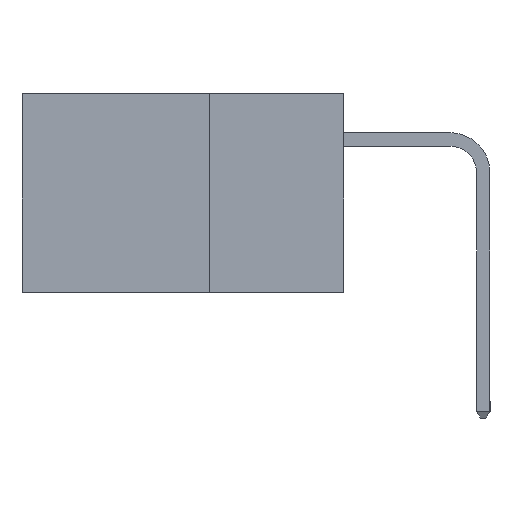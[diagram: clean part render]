
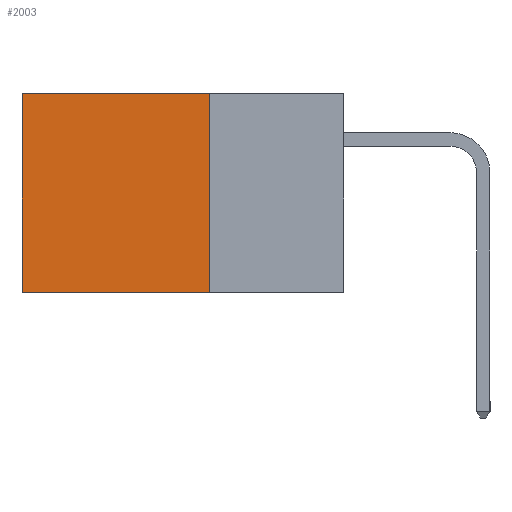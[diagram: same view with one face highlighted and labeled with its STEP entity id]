
A CAD part, left-side view. The second image highlights one B-rep face of the part: STEP entity #2003.
In plain terms, the highlighted planar face has unit normal (-1, 0, 0).
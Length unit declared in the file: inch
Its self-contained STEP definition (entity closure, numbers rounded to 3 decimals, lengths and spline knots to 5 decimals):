
#480 = VECTOR ( 'NONE', #2758, 39.37008 ) ;
#621 = CARTESIAN_POINT ( 'NONE',  ( 0.2615, 0.25, -0.37 ) ) ;
#810 = LINE ( 'NONE', #5589, #8700 ) ;
#1602 = EDGE_CURVE ( 'NONE', #5127, #11629, #3533, .T. ) ;
#2003 = ADVANCED_FACE ( 'NONE', ( #2388 ), #10919, .F. ) ;
#2063 = CARTESIAN_POINT ( 'NONE',  ( 0.2615, 0.25, 0. ) ) ;
#2388 = FACE_OUTER_BOUND ( 'NONE', #12728, .T. ) ;
#2590 = VERTEX_POINT ( 'NONE', #5535 ) ;
#2758 = DIRECTION ( 'NONE',  ( 0., 0., -1. ) ) ;
#3533 = LINE ( 'NONE', #10657, #480 ) ;
#5127 = VERTEX_POINT ( 'NONE', #14093 ) ;
#5492 = LINE ( 'NONE', #2063, #12486 ) ;
#5535 = CARTESIAN_POINT ( 'NONE',  ( 0.2615, 0.6, 0. ) ) ;
#5589 = CARTESIAN_POINT ( 'NONE',  ( 0.2615, 0.25, -0.37 ) ) ;
#5683 = ORIENTED_EDGE ( 'NONE', *, *, #10510, .T. ) ;
#6492 = CARTESIAN_POINT ( 'NONE',  ( 0.2615, 0.25, -0.37 ) ) ;
#6732 = DIRECTION ( 'NONE',  ( 0., 1., 0. ) ) ;
#7025 = DIRECTION ( 'NONE',  ( 0., 0., -1. ) ) ;
#7099 = DIRECTION ( 'NONE',  ( 1., 0., 0. ) ) ;
#7824 = ORIENTED_EDGE ( 'NONE', *, *, #10546, .F. ) ;
#8700 = VECTOR ( 'NONE', #10100, 39.37008 ) ;
#8756 = ORIENTED_EDGE ( 'NONE', *, *, #9602, .T. ) ;
#9108 = LINE ( 'NONE', #11697, #14690 ) ;
#9436 = DIRECTION ( 'NONE',  ( 0., 0., -1. ) ) ;
#9602 = EDGE_CURVE ( 'NONE', #2590, #11001, #9108, .T. ) ;
#10100 = DIRECTION ( 'NONE',  ( 0., 1., 0. ) ) ;
#10420 = ORIENTED_EDGE ( 'NONE', *, *, #1602, .F. ) ;
#10510 = EDGE_CURVE ( 'NONE', #5127, #2590, #5492, .T. ) ;
#10546 = EDGE_CURVE ( 'NONE', #11629, #11001, #810, .T. ) ;
#10608 = AXIS2_PLACEMENT_3D ( 'NONE', #621, #7099, #7025 ) ;
#10657 = CARTESIAN_POINT ( 'NONE',  ( 0.2615, 0.25, -0.37 ) ) ;
#10919 = PLANE ( 'NONE',  #10608 ) ;
#11001 = VERTEX_POINT ( 'NONE', #14383 ) ;
#11629 = VERTEX_POINT ( 'NONE', #6492 ) ;
#11697 = CARTESIAN_POINT ( 'NONE',  ( 0.2615, 0.6, -0.37 ) ) ;
#12486 = VECTOR ( 'NONE', #6732, 39.37008 ) ;
#12728 = EDGE_LOOP ( 'NONE', ( #8756, #7824, #10420, #5683 ) ) ;
#14093 = CARTESIAN_POINT ( 'NONE',  ( 0.2615, 0.25, 0. ) ) ;
#14383 = CARTESIAN_POINT ( 'NONE',  ( 0.2615, 0.6, -0.37 ) ) ;
#14690 = VECTOR ( 'NONE', #9436, 39.37008 ) ;
